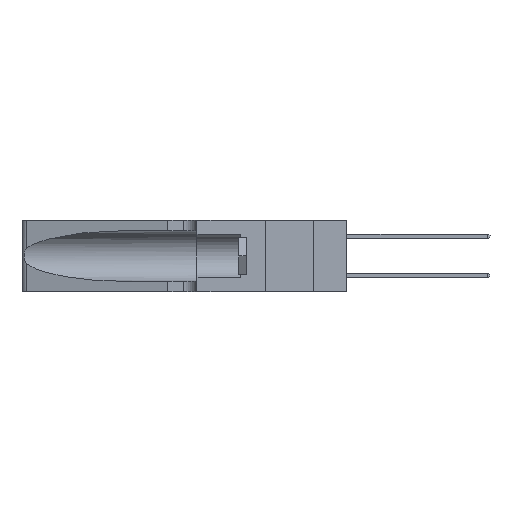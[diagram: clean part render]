
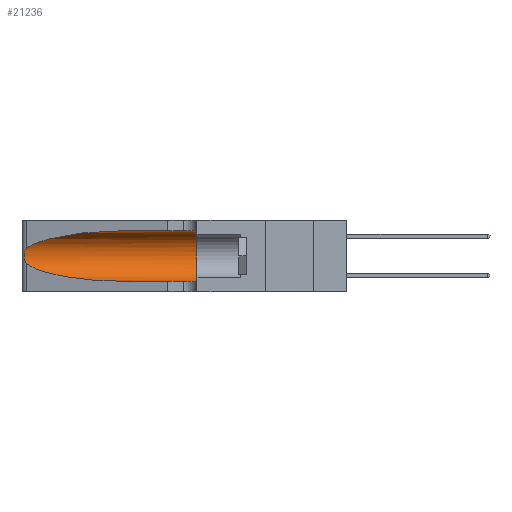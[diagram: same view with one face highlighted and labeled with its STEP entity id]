
A CAD part, left-side view. The second image highlights one B-rep face of the part: STEP entity #21236.
In plain terms, the highlighted cylindrical face has radius 3.308 mm (diameter 6.617 mm), a partial arc.
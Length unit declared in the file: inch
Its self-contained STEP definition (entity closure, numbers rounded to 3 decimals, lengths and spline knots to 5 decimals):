
#1254 = CARTESIAN_POINT ( 'NONE',  ( 0.26018, 1.23835, 0.19895 ) ) ;
#1352 = DIRECTION ( 'NONE',  ( 0., -1., 0. ) ) ;
#1813 = CARTESIAN_POINT ( 'NONE',  ( 0.25555, 1.22993, 0.14849 ) ) ;
#2267 = CARTESIAN_POINT ( 'NONE',  ( 0.1305, 0.35, 0.31525 ) ) ;
#3352 = FACE_OUTER_BOUND ( 'NONE', #26726, .T. ) ;
#3489 = AXIS2_PLACEMENT_3D ( 'NONE', #14135, #1352, #24706 ) ;
#3865 = ORIENTED_EDGE ( 'NONE', *, *, #29753, .F. ) ;
#4477 = CARTESIAN_POINT ( 'NONE',  ( 0.26075, 1.23896, 0.178 ) ) ;
#4824 = LINE ( 'NONE', #16692, #18470 ) ;
#5319 = CARTESIAN_POINT ( 'NONE',  ( 0.25639, 1.23186, 0.15144 ) ) ;
#6892 = ORIENTED_EDGE ( 'NONE', *, *, #25008, .T. ) ;
#7074 =( BOUNDED_CURVE ( )  B_SPLINE_CURVE ( 3, ( #7310, #36077, #7444, #10712 ),
 .UNSPECIFIED., .F., .T. ) 
 B_SPLINE_CURVE_WITH_KNOTS ( ( 4, 4 ),
 ( 1.5708, 2.84003 ),
 .UNSPECIFIED. ) 
 CURVE ( )  GEOMETRIC_REPRESENTATION_ITEM ( )  RATIONAL_B_SPLINE_CURVE ( ( 1., 0.87, 0.87, 1. ) ) 
 REPRESENTATION_ITEM ( '' )  );
#7213 = EDGE_CURVE ( 'NONE', #18986, #12886, #14664, .T. ) ;
#7310 = CARTESIAN_POINT ( 'NONE',  ( 0.1305, 0.72297, 0.31525 ) ) ;
#7444 = CARTESIAN_POINT ( 'NONE',  ( 0.2373, 1.15595, 0.28018 ) ) ;
#9570 = CARTESIAN_POINT ( 'NONE',  ( 0.1305, 0.72297, 0.31525 ) ) ;
#10093 = CARTESIAN_POINT ( 'NONE',  ( 0.1305, 0.72297, 0.05475 ) ) ;
#10712 = CARTESIAN_POINT ( 'NONE',  ( 0.25487, 1.22718, 0.22369 ) ) ;
#11624 = CARTESIAN_POINT ( 'NONE',  ( 0.25487, 1.22718, 0.14631 ) ) ;
#12886 = VERTEX_POINT ( 'NONE', #36162 ) ;
#12967 = CARTESIAN_POINT ( 'NONE',  ( 0.25487, 1.22718, 0.14631 ) ) ;
#13028 = CARTESIAN_POINT ( 'NONE',  ( 0.25487, 1.22718, 0.22369 ) ) ;
#13104 = CARTESIAN_POINT ( 'NONE',  ( 0.18966, 0.96281, 0.05475 ) ) ;
#13551 = VERTEX_POINT ( 'NONE', #2267 ) ;
#14053 = CARTESIAN_POINT ( 'NONE',  ( 0.25787, 1.23484, 0.2124 ) ) ;
#14135 = CARTESIAN_POINT ( 'NONE',  ( 0.1305, 1.61858, 0.185 ) ) ;
#14664 =( BOUNDED_CURVE ( )  B_SPLINE_CURVE ( 3, ( #12967, #38995, #13104, #10093 ),
 .UNSPECIFIED., .F., .F. ) 
 B_SPLINE_CURVE_WITH_KNOTS ( ( 4, 4 ),
 ( 3.44316, 4.71239 ),
 .UNSPECIFIED. ) 
 CURVE ( )  GEOMETRIC_REPRESENTATION_ITEM ( )  RATIONAL_B_SPLINE_CURVE ( ( 1., 0.87, 0.87, 1. ) ) 
 REPRESENTATION_ITEM ( '' )  );
#15722 = CARTESIAN_POINT ( 'NONE',  ( 0.1305, 0.35, 0.05475 ) ) ;
#16692 = CARTESIAN_POINT ( 'NONE',  ( 0.1305, 1.61858, 0.31525 ) ) ;
#16914 = AXIS2_PLACEMENT_3D ( 'NONE', #23429, #30043, #26518 ) ;
#17748 = CARTESIAN_POINT ( 'NONE',  ( 0.25487, 1.22718, 0.22369 ) ) ;
#18185 = VERTEX_POINT ( 'NONE', #15722 ) ;
#18470 = VECTOR ( 'NONE', #26536, 39.37008 ) ;
#18953 = EDGE_CURVE ( 'NONE', #12886, #18185, #20695, .T. ) ;
#18986 = VERTEX_POINT ( 'NONE', #30117 ) ;
#19645 = ORIENTED_EDGE ( 'NONE', *, *, #18953, .T. ) ;
#20695 = LINE ( 'NONE', #32649, #33768 ) ;
#21125 = B_SPLINE_CURVE_WITH_KNOTS ( 'NONE', 3,
 ( #17748, #33199, #23625, #14053, #30248, #1254, #36560, #4477, #26998, #33488, #39920, #5319, #1813, #11624 ),
 .UNSPECIFIED., .F., .F.,
 ( 4, 2, 2, 2, 2, 2, 4 ),
 ( 0., 0.00027, 0.00053, 0.00107, 0.0016, 0.00187, 0.00214 ),
 .UNSPECIFIED. ) ;
#21157 = EDGE_CURVE ( 'NONE', #35712, #38754, #7074, .T. ) ;
#21236 = ADVANCED_FACE ( 'NONE', ( #3352 ), #29097, .F. ) ;
#23075 = DIRECTION ( 'NONE',  ( 0., -1., 0. ) ) ;
#23429 = CARTESIAN_POINT ( 'NONE',  ( 0.1305, 0.35, 0.185 ) ) ;
#23625 = CARTESIAN_POINT ( 'NONE',  ( 0.25639, 1.23184, 0.21858 ) ) ;
#24706 = DIRECTION ( 'NONE',  ( 0., 0., -1. ) ) ;
#25008 = EDGE_CURVE ( 'NONE', #38754, #18986, #21125, .T. ) ;
#26518 = DIRECTION ( 'NONE',  ( 0., 0., 1. ) ) ;
#26536 = DIRECTION ( 'NONE',  ( 0., -1., 0. ) ) ;
#26726 = EDGE_LOOP ( 'NONE', ( #38862, #6892, #33288, #19645, #3865, #35046 ) ) ;
#26998 = CARTESIAN_POINT ( 'NONE',  ( 0.26017, 1.23833, 0.17102 ) ) ;
#29097 = CYLINDRICAL_SURFACE ( 'NONE', #3489, 0.13025 ) ;
#29753 = EDGE_CURVE ( 'NONE', #13551, #18185, #40818, .T. ) ;
#30043 = DIRECTION ( 'NONE',  ( 0., 1., 0. ) ) ;
#30117 = CARTESIAN_POINT ( 'NONE',  ( 0.25487, 1.22718, 0.14631 ) ) ;
#30248 = CARTESIAN_POINT ( 'NONE',  ( 0.25854, 1.2359, 0.20912 ) ) ;
#32649 = CARTESIAN_POINT ( 'NONE',  ( 0.1305, 1.61858, 0.05475 ) ) ;
#33199 = CARTESIAN_POINT ( 'NONE',  ( 0.25555, 1.22994, 0.2215 ) ) ;
#33288 = ORIENTED_EDGE ( 'NONE', *, *, #7213, .T. ) ;
#33488 = CARTESIAN_POINT ( 'NONE',  ( 0.25856, 1.23593, 0.16098 ) ) ;
#33768 = VECTOR ( 'NONE', #23075, 39.37008 ) ;
#35046 = ORIENTED_EDGE ( 'NONE', *, *, #35170, .F. ) ;
#35170 = EDGE_CURVE ( 'NONE', #35712, #13551, #4824, .T. ) ;
#35712 = VERTEX_POINT ( 'NONE', #9570 ) ;
#36077 = CARTESIAN_POINT ( 'NONE',  ( 0.18966, 0.96281, 0.31525 ) ) ;
#36162 = CARTESIAN_POINT ( 'NONE',  ( 0.1305, 0.72297, 0.05475 ) ) ;
#36560 = CARTESIAN_POINT ( 'NONE',  ( 0.26075, 1.23896, 0.19203 ) ) ;
#38754 = VERTEX_POINT ( 'NONE', #13028 ) ;
#38862 = ORIENTED_EDGE ( 'NONE', *, *, #21157, .T. ) ;
#38995 = CARTESIAN_POINT ( 'NONE',  ( 0.2373, 1.15595, 0.08982 ) ) ;
#39920 = CARTESIAN_POINT ( 'NONE',  ( 0.25789, 1.23486, 0.15765 ) ) ;
#40818 = CIRCLE ( 'NONE', #16914, 0.13025 ) ;
